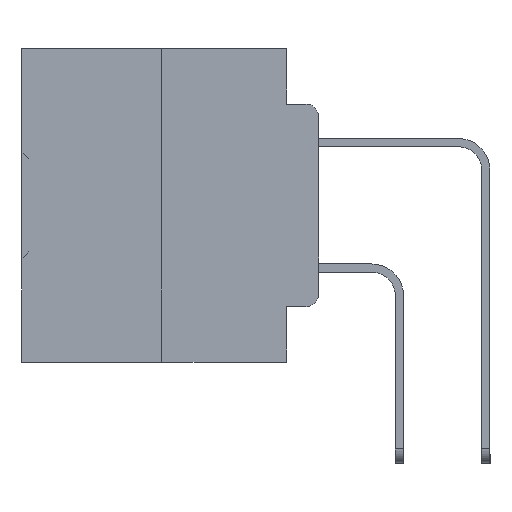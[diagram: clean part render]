
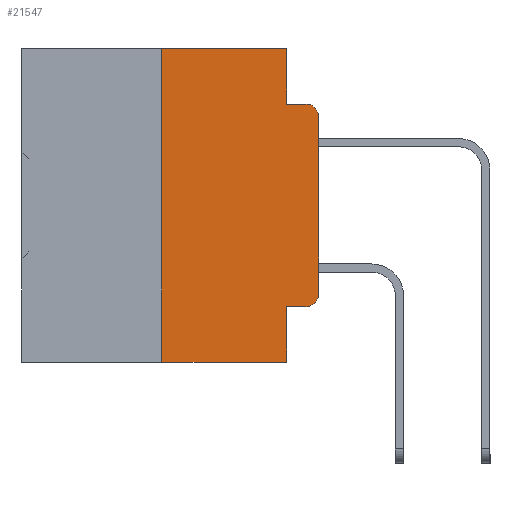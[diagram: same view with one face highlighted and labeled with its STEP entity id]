
A CAD part, left-side view. The second image highlights one B-rep face of the part: STEP entity #21547.
In plain terms, the highlighted planar face has unit normal (-1, 0, 0).
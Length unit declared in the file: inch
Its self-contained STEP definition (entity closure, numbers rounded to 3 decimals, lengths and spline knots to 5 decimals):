
#20 = EDGE_CURVE ( 'NONE', #37751, #35358, #26989, .T. ) ;
#520 = LINE ( 'NONE', #27398, #31486 ) ;
#2074 = EDGE_CURVE ( 'NONE', #27134, #37751, #28201, .T. ) ;
#2631 = FACE_OUTER_BOUND ( 'NONE', #28726, .T. ) ;
#2952 = DIRECTION ( 'NONE',  ( 0., -1., 0. ) ) ;
#3980 = ORIENTED_EDGE ( 'NONE', *, *, #14463, .F. ) ;
#4273 = CARTESIAN_POINT ( 'NONE',  ( 0., 0.051, 0. ) ) ;
#4477 = LINE ( 'NONE', #22144, #27422 ) ;
#5521 = DIRECTION ( 'NONE',  ( -1., 0., 0. ) ) ;
#5861 = DIRECTION ( 'NONE',  ( 1., 0., 0. ) ) ;
#6022 = EDGE_CURVE ( 'NONE', #15990, #24839, #4477, .T. ) ;
#7039 = DIRECTION ( 'NONE',  ( 0., -1., 0. ) ) ;
#7108 = EDGE_CURVE ( 'NONE', #12719, #21563, #520, .T. ) ;
#7705 = DIRECTION ( 'NONE',  ( 0., 0., -1. ) ) ;
#7832 = CARTESIAN_POINT ( 'NONE',  ( 0., 0.051, -0.5 ) ) ;
#8095 = LINE ( 'NONE', #4273, #29906 ) ;
#8397 = CARTESIAN_POINT ( 'NONE',  ( 0., 0., 0. ) ) ;
#9407 = ORIENTED_EDGE ( 'NONE', *, *, #34174, .T. ) ;
#10448 = EDGE_CURVE ( 'NONE', #27134, #24839, #8095, .T. ) ;
#10691 = DIRECTION ( 'NONE',  ( 0., -1., 0. ) ) ;
#10829 = VECTOR ( 'NONE', #10691, 39.37008 ) ;
#12385 = CARTESIAN_POINT ( 'NONE',  ( 0., 0.051, -0.4115 ) ) ;
#12460 = EDGE_CURVE ( 'NONE', #15990, #12719, #31940, .T. ) ;
#12719 = VERTEX_POINT ( 'NONE', #32296 ) ;
#12722 = CIRCLE ( 'NONE', #17658, 0.02 ) ;
#13658 = CARTESIAN_POINT ( 'NONE',  ( 0., 0.02, -0.0885 ) ) ;
#14463 = EDGE_CURVE ( 'NONE', #21563, #25424, #23139, .T. ) ;
#14910 = AXIS2_PLACEMENT_3D ( 'NONE', #37914, #20053, #25115 ) ;
#15506 = ORIENTED_EDGE ( 'NONE', *, *, #24366, .T. ) ;
#15541 = ORIENTED_EDGE ( 'NONE', *, *, #2074, .T. ) ;
#15990 = VERTEX_POINT ( 'NONE', #35654 ) ;
#16678 = DIRECTION ( 'NONE',  ( 0., 0., 1. ) ) ;
#16813 = CARTESIAN_POINT ( 'NONE',  ( 0., 0.051, -0.0885 ) ) ;
#17658 = AXIS2_PLACEMENT_3D ( 'NONE', #23551, #5521, #26463 ) ;
#17811 = CARTESIAN_POINT ( 'NONE',  ( 0., 0.02, -0.4115 ) ) ;
#17878 = LINE ( 'NONE', #8397, #25619 ) ;
#18740 = DIRECTION ( 'NONE',  ( 0., -1., 0. ) ) ;
#19574 = CARTESIAN_POINT ( 'NONE',  ( 0., 0.051, 0. ) ) ;
#20053 = DIRECTION ( 'NONE',  ( -1., 0., 0. ) ) ;
#20171 = CARTESIAN_POINT ( 'NONE',  ( 0., 0., -0.1085 ) ) ;
#20526 = AXIS2_PLACEMENT_3D ( 'NONE', #32581, #5861, #26769 ) ;
#20941 = PLANE ( 'NONE',  #20526 ) ;
#21547 = ADVANCED_FACE ( 'NONE', ( #2631 ), #20941, .F. ) ;
#21563 = VERTEX_POINT ( 'NONE', #23987 ) ;
#22144 = CARTESIAN_POINT ( 'NONE',  ( 0., 0.473, -0.5 ) ) ;
#22387 = DIRECTION ( 'NONE',  ( 0., 0., -1. ) ) ;
#22409 = EDGE_CURVE ( 'NONE', #25424, #26823, #26552, .T. ) ;
#23139 = LINE ( 'NONE', #19574, #37854 ) ;
#23551 = CARTESIAN_POINT ( 'NONE',  ( 0., 0.02, -0.1085 ) ) ;
#23987 = CARTESIAN_POINT ( 'NONE',  ( 0., 0.051, 0. ) ) ;
#24366 = EDGE_CURVE ( 'NONE', #29197, #26823, #12722, .T. ) ;
#24839 = VERTEX_POINT ( 'NONE', #7832 ) ;
#25115 = DIRECTION ( 'NONE',  ( 0., 0., -1. ) ) ;
#25424 = VERTEX_POINT ( 'NONE', #16813 ) ;
#25439 = CARTESIAN_POINT ( 'NONE',  ( 0., 0.051, -0.0885 ) ) ;
#25619 = VECTOR ( 'NONE', #29118, 39.37008 ) ;
#26463 = DIRECTION ( 'NONE',  ( 0., 0., -1. ) ) ;
#26536 = ORIENTED_EDGE ( 'NONE', *, *, #6022, .T. ) ;
#26552 = LINE ( 'NONE', #25439, #10829 ) ;
#26769 = DIRECTION ( 'NONE',  ( 0., 0., -1. ) ) ;
#26823 = VERTEX_POINT ( 'NONE', #13658 ) ;
#26989 = CIRCLE ( 'NONE', #14910, 0.02 ) ;
#27134 = VERTEX_POINT ( 'NONE', #32808 ) ;
#27268 = VECTOR ( 'NONE', #2952, 39.37008 ) ;
#27398 = CARTESIAN_POINT ( 'NONE',  ( 0., 0.473, 0. ) ) ;
#27422 = VECTOR ( 'NONE', #7039, 39.37008 ) ;
#28201 = LINE ( 'NONE', #12385, #27268 ) ;
#28461 = CARTESIAN_POINT ( 'NONE',  ( 0., 0., -0.3915 ) ) ;
#28726 = EDGE_LOOP ( 'NONE', ( #9407, #15506, #31090, #3980, #38539, #32526, #26536, #38096, #15541, #33000 ) ) ;
#29118 = DIRECTION ( 'NONE',  ( 0., 0., 1. ) ) ;
#29197 = VERTEX_POINT ( 'NONE', #20171 ) ;
#29906 = VECTOR ( 'NONE', #22387, 39.37008 ) ;
#30083 = VECTOR ( 'NONE', #16678, 39.37008 ) ;
#31090 = ORIENTED_EDGE ( 'NONE', *, *, #22409, .F. ) ;
#31257 = CARTESIAN_POINT ( 'NONE',  ( 0., 0.25, 0. ) ) ;
#31486 = VECTOR ( 'NONE', #18740, 39.37008 ) ;
#31940 = LINE ( 'NONE', #31257, #30083 ) ;
#32296 = CARTESIAN_POINT ( 'NONE',  ( 0., 0.25, 0. ) ) ;
#32526 = ORIENTED_EDGE ( 'NONE', *, *, #12460, .F. ) ;
#32581 = CARTESIAN_POINT ( 'NONE',  ( 0., 0.473, 0. ) ) ;
#32808 = CARTESIAN_POINT ( 'NONE',  ( 0., 0.051, -0.4115 ) ) ;
#33000 = ORIENTED_EDGE ( 'NONE', *, *, #20, .T. ) ;
#34174 = EDGE_CURVE ( 'NONE', #35358, #29197, #17878, .T. ) ;
#35358 = VERTEX_POINT ( 'NONE', #28461 ) ;
#35654 = CARTESIAN_POINT ( 'NONE',  ( 0., 0.25, -0.5 ) ) ;
#37751 = VERTEX_POINT ( 'NONE', #17811 ) ;
#37854 = VECTOR ( 'NONE', #7705, 39.37008 ) ;
#37914 = CARTESIAN_POINT ( 'NONE',  ( 0., 0.02, -0.3915 ) ) ;
#38096 = ORIENTED_EDGE ( 'NONE', *, *, #10448, .F. ) ;
#38539 = ORIENTED_EDGE ( 'NONE', *, *, #7108, .F. ) ;
